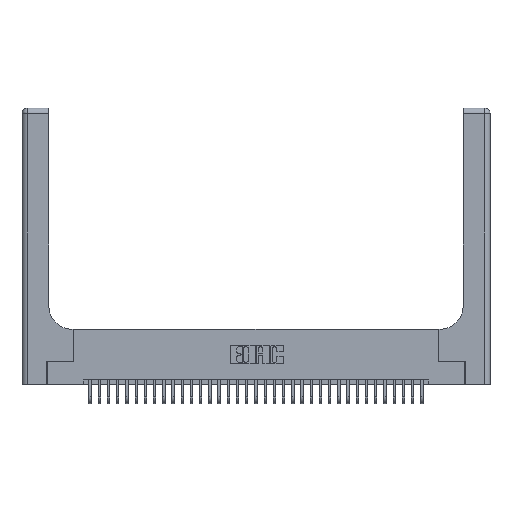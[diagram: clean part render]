
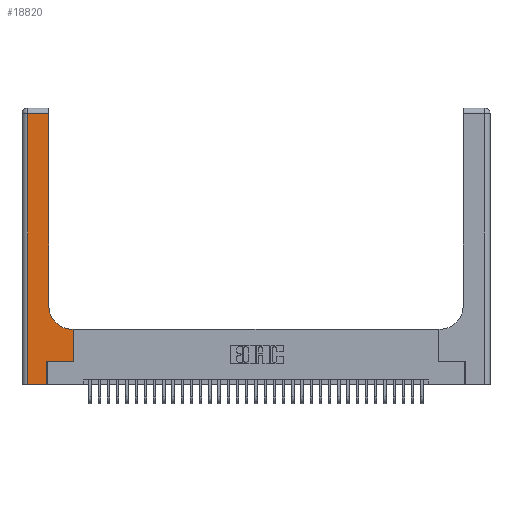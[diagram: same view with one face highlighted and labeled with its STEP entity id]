
A CAD part, top view. The second image highlights one B-rep face of the part: STEP entity #18820.
In plain terms, the highlighted planar face has unit normal (0, 0, 1).
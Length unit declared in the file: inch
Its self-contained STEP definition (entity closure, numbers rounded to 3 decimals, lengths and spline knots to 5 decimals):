
#325 = LINE ( 'NONE', #6553, #23293 ) ;
#1299 = VECTOR ( 'NONE', #28802, 39.37008 ) ;
#2056 = CARTESIAN_POINT ( 'NONE',  ( 0.06, 0., 0.37 ) ) ;
#2278 = ORIENTED_EDGE ( 'NONE', *, *, #34425, .T. ) ;
#2455 = EDGE_CURVE ( 'NONE', #11930, #10262, #7283, .T. ) ;
#2541 = CARTESIAN_POINT ( 'NONE',  ( 0., 3., 0.37 ) ) ;
#2714 = VECTOR ( 'NONE', #19476, 39.37008 ) ;
#3241 = EDGE_CURVE ( 'NONE', #31462, #31741, #28779, .T. ) ;
#3952 = ORIENTED_EDGE ( 'NONE', *, *, #18449, .T. ) ;
#4332 = CARTESIAN_POINT ( 'NONE',  ( 0.269, 0.25, 0.37 ) ) ;
#4885 = LINE ( 'NONE', #5271, #32678 ) ;
#5271 = CARTESIAN_POINT ( 'NONE',  ( 0.269, 0.25, 0.37 ) ) ;
#6098 = CARTESIAN_POINT ( 'NONE',  ( 0.269, 0., 0.37 ) ) ;
#6289 = VECTOR ( 'NONE', #35080, 39.37008 ) ;
#6524 = VECTOR ( 'NONE', #28008, 39.37008 ) ;
#6553 = CARTESIAN_POINT ( 'NONE',  ( 0.06, 3., 0.37 ) ) ;
#6941 = EDGE_CURVE ( 'NONE', #11115, #31462, #325, .T. ) ;
#7108 = ORIENTED_EDGE ( 'NONE', *, *, #2455, .T. ) ;
#7162 = LINE ( 'NONE', #29901, #21262 ) ;
#7283 = CIRCLE ( 'NONE', #22633, 0.25 ) ;
#8114 = DIRECTION ( 'NONE',  ( -1., 0., 0. ) ) ;
#8167 = ORIENTED_EDGE ( 'NONE', *, *, #3241, .T. ) ;
#8436 = EDGE_CURVE ( 'NONE', #31741, #16736, #29014, .T. ) ;
#9320 = EDGE_CURVE ( 'NONE', #33210, #10412, #20079, .T. ) ;
#9366 = ORIENTED_EDGE ( 'NONE', *, *, #14477, .T. ) ;
#10262 = VERTEX_POINT ( 'NONE', #14976 ) ;
#10412 = VERTEX_POINT ( 'NONE', #27927 ) ;
#11115 = VERTEX_POINT ( 'NONE', #36098 ) ;
#11930 = VERTEX_POINT ( 'NONE', #30121 ) ;
#12644 = VECTOR ( 'NONE', #28092, 39.37008 ) ;
#13855 = CARTESIAN_POINT ( 'NONE',  ( 0.269, 0., 0.37 ) ) ;
#13924 = DIRECTION ( 'NONE',  ( 0., 0., -1. ) ) ;
#14477 = EDGE_CURVE ( 'NONE', #10262, #20371, #20720, .T. ) ;
#14976 = CARTESIAN_POINT ( 'NONE',  ( 0.2915, 0.85, 0.37 ) ) ;
#16736 = VERTEX_POINT ( 'NONE', #4332 ) ;
#16875 = DIRECTION ( 'NONE',  ( -1., 0., 0. ) ) ;
#17692 = LINE ( 'NONE', #33102, #2714 ) ;
#18272 = DIRECTION ( 'NONE',  ( 0., -1., 0. ) ) ;
#18449 = EDGE_CURVE ( 'NONE', #10412, #11930, #17692, .T. ) ;
#18592 = EDGE_LOOP ( 'NONE', ( #9366, #32596, #22919, #8167, #21882, #2278, #26452, #3952, #7108 ) ) ;
#18820 = ADVANCED_FACE ( 'NONE', ( #23129 ), #19433, .F. ) ;
#19433 = PLANE ( 'NONE',  #27933 ) ;
#19476 = DIRECTION ( 'NONE',  ( -1., 0., 0. ) ) ;
#20079 = LINE ( 'NONE', #28324, #12644 ) ;
#20298 = DIRECTION ( 'NONE',  ( 0., 0., -1. ) ) ;
#20371 = VERTEX_POINT ( 'NONE', #30031 ) ;
#20720 = LINE ( 'NONE', #23013, #1299 ) ;
#21262 = VECTOR ( 'NONE', #8114, 39.37008 ) ;
#21882 = ORIENTED_EDGE ( 'NONE', *, *, #8436, .T. ) ;
#22633 = AXIS2_PLACEMENT_3D ( 'NONE', #34399, #20298, #31682 ) ;
#22919 = ORIENTED_EDGE ( 'NONE', *, *, #6941, .T. ) ;
#22958 = CARTESIAN_POINT ( 'NONE',  ( 0.5585, 0.25, 0.37 ) ) ;
#23013 = CARTESIAN_POINT ( 'NONE',  ( 0.2915, 3., 0.37 ) ) ;
#23129 = FACE_OUTER_BOUND ( 'NONE', #18592, .T. ) ;
#23293 = VECTOR ( 'NONE', #18272, 39.37008 ) ;
#24779 = DIRECTION ( 'NONE',  ( 1., 0., 0. ) ) ;
#26452 = ORIENTED_EDGE ( 'NONE', *, *, #9320, .T. ) ;
#27927 = CARTESIAN_POINT ( 'NONE',  ( 0.5585, 0.6, 0.37 ) ) ;
#27933 = AXIS2_PLACEMENT_3D ( 'NONE', #2541, #13924, #16875 ) ;
#28008 = DIRECTION ( 'NONE',  ( 0., 1., 0. ) ) ;
#28092 = DIRECTION ( 'NONE',  ( 0., 1., 0. ) ) ;
#28324 = CARTESIAN_POINT ( 'NONE',  ( 0.5585, 0.25, 0.37 ) ) ;
#28752 = CARTESIAN_POINT ( 'NONE',  ( 0., 0., 0.37 ) ) ;
#28779 = LINE ( 'NONE', #28752, #6289 ) ;
#28802 = DIRECTION ( 'NONE',  ( 0., 1., 0. ) ) ;
#29014 = LINE ( 'NONE', #13855, #6524 ) ;
#29901 = CARTESIAN_POINT ( 'NONE',  ( 0., 2.94, 0.37 ) ) ;
#30031 = CARTESIAN_POINT ( 'NONE',  ( 0.2915, 2.94, 0.37 ) ) ;
#30121 = CARTESIAN_POINT ( 'NONE',  ( 0.5415, 0.6, 0.37 ) ) ;
#31462 = VERTEX_POINT ( 'NONE', #2056 ) ;
#31682 = DIRECTION ( 'NONE',  ( 1., 0., 0. ) ) ;
#31741 = VERTEX_POINT ( 'NONE', #6098 ) ;
#32596 = ORIENTED_EDGE ( 'NONE', *, *, #33065, .T. ) ;
#32678 = VECTOR ( 'NONE', #24779, 39.37008 ) ;
#33065 = EDGE_CURVE ( 'NONE', #20371, #11115, #7162, .T. ) ;
#33102 = CARTESIAN_POINT ( 'NONE',  ( 0.2915, 0.6, 0.37 ) ) ;
#33210 = VERTEX_POINT ( 'NONE', #22958 ) ;
#34399 = CARTESIAN_POINT ( 'NONE',  ( 0.5415, 0.85, 0.37 ) ) ;
#34425 = EDGE_CURVE ( 'NONE', #16736, #33210, #4885, .T. ) ;
#35080 = DIRECTION ( 'NONE',  ( 1., 0., 0. ) ) ;
#36098 = CARTESIAN_POINT ( 'NONE',  ( 0.06, 2.94, 0.37 ) ) ;
